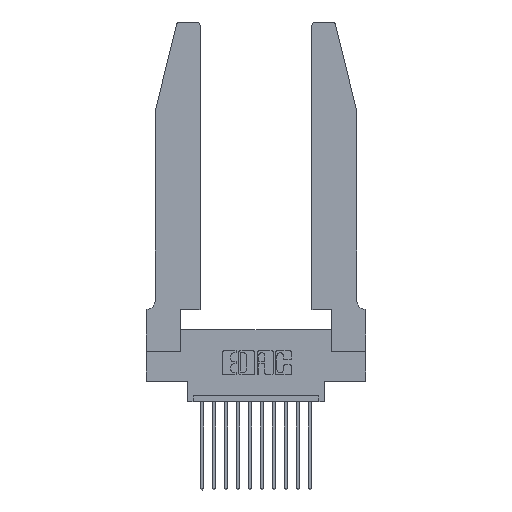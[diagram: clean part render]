
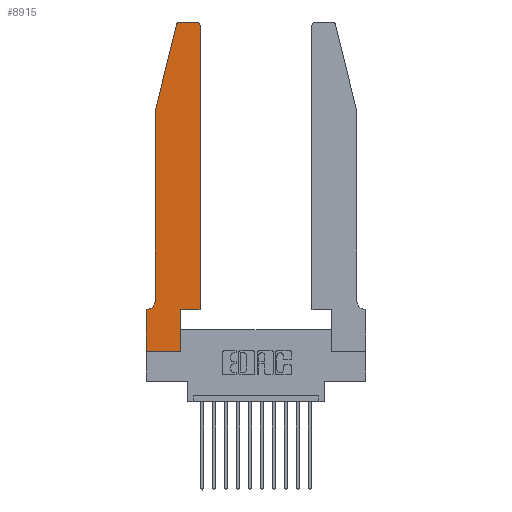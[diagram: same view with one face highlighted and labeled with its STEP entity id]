
A CAD part, top view. The second image highlights one B-rep face of the part: STEP entity #8915.
In plain terms, the highlighted planar face has unit normal (0, 0, 1).
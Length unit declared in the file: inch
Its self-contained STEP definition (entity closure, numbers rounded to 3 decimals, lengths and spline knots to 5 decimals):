
#252 = DIRECTION ( 'NONE',  ( 1., 0., 0. ) ) ;
#673 = VERTEX_POINT ( 'NONE', #13851 ) ;
#1145 = CARTESIAN_POINT ( 'NONE',  ( 0.25487, 2.72718, 0.37 ) ) ;
#1256 = CARTESIAN_POINT ( 'NONE',  ( 0.2865, 0.35, 0.37 ) ) ;
#1277 = DIRECTION ( 'NONE',  ( -1., 0., 0. ) ) ;
#1287 = CARTESIAN_POINT ( 'NONE',  ( 0.4505, 0.35, 0.37 ) ) ;
#1292 = EDGE_CURVE ( 'NONE', #7875, #4004, #4837, .T. ) ;
#1612 = CIRCLE ( 'NONE', #16716, 0.03 ) ;
#1732 = CARTESIAN_POINT ( 'NONE',  ( 0., 0.35, 0.37 ) ) ;
#1873 = VECTOR ( 'NONE', #9829, 39.37008 ) ;
#1878 = DIRECTION ( 'NONE',  ( 0., 0., 1. ) ) ;
#1887 = CARTESIAN_POINT ( 'NONE',  ( 0.284, 2.75, 0.37 ) ) ;
#2018 = VECTOR ( 'NONE', #13395, 39.37008 ) ;
#2041 = CARTESIAN_POINT ( 'NONE',  ( 0., 0.35, 0.37 ) ) ;
#2090 = VECTOR ( 'NONE', #2855, 39.37008 ) ;
#2194 = DIRECTION ( 'NONE',  ( -1., 0., 0. ) ) ;
#2246 = AXIS2_PLACEMENT_3D ( 'NONE', #15536, #1878, #14213 ) ;
#2300 = VERTEX_POINT ( 'NONE', #8853 ) ;
#2461 = VERTEX_POINT ( 'NONE', #11688 ) ;
#2654 = ORIENTED_EDGE ( 'NONE', *, *, #15632, .T. ) ;
#2749 = VECTOR ( 'NONE', #9596, 39.37008 ) ;
#2855 = DIRECTION ( 'NONE',  ( 1., 0., 0. ) ) ;
#2965 = EDGE_CURVE ( 'NONE', #9443, #16137, #1612, .T. ) ;
#3316 = CARTESIAN_POINT ( 'NONE',  ( 0.284, 2.72, 0.37 ) ) ;
#3427 = CARTESIAN_POINT ( 'NONE',  ( 0.0755, 2., 0.37 ) ) ;
#3888 = LINE ( 'NONE', #3427, #4703 ) ;
#4004 = VERTEX_POINT ( 'NONE', #6656 ) ;
#4189 = CARTESIAN_POINT ( 'NONE',  ( 0.0755, 2., 0.37 ) ) ;
#4335 = VERTEX_POINT ( 'NONE', #2041 ) ;
#4581 = EDGE_CURVE ( 'NONE', #13725, #2461, #10868, .T. ) ;
#4646 = CARTESIAN_POINT ( 'NONE',  ( 0.0755, 2., 0.37 ) ) ;
#4698 = DIRECTION ( 'NONE',  ( 0., 1., 0. ) ) ;
#4703 = VECTOR ( 'NONE', #10340, 39.37008 ) ;
#4837 = LINE ( 'NONE', #12212, #2018 ) ;
#4920 = ORIENTED_EDGE ( 'NONE', *, *, #13394, .T. ) ;
#5031 = VECTOR ( 'NONE', #9676, 39.37008 ) ;
#5240 = VERTEX_POINT ( 'NONE', #4189 ) ;
#5259 = AXIS2_PLACEMENT_3D ( 'NONE', #15546, #15660, #1277 ) ;
#5414 = LINE ( 'NONE', #12222, #5031 ) ;
#5914 = ORIENTED_EDGE ( 'NONE', *, *, #1292, .T. ) ;
#6072 = ORIENTED_EDGE ( 'NONE', *, *, #6856, .T. ) ;
#6265 = ORIENTED_EDGE ( 'NONE', *, *, #4581, .T. ) ;
#6473 = EDGE_CURVE ( 'NONE', #16137, #5240, #9374, .T. ) ;
#6656 = CARTESIAN_POINT ( 'NONE',  ( 0.2865, 0., 0.37 ) ) ;
#6856 = EDGE_CURVE ( 'NONE', #2300, #15438, #7971, .T. ) ;
#6866 = PLANE ( 'NONE',  #12857 ) ;
#7240 = CARTESIAN_POINT ( 'NONE',  ( 0., 0., 0.37 ) ) ;
#7875 = VERTEX_POINT ( 'NONE', #11843 ) ;
#7971 = CIRCLE ( 'NONE', #5259, 0.07 ) ;
#7999 = DIRECTION ( 'NONE',  ( 0., 0., 1. ) ) ;
#8172 = LINE ( 'NONE', #1256, #15443 ) ;
#8765 = LINE ( 'NONE', #7240, #1873 ) ;
#8788 = EDGE_LOOP ( 'NONE', ( #10304, #10822, #11894, #16695, #6072, #16342, #10317, #5914, #16578, #4920, #6265, #2654 ) ) ;
#8853 = CARTESIAN_POINT ( 'NONE',  ( 0.0755, 0.42, 0.37 ) ) ;
#8915 = ADVANCED_FACE ( 'NONE', ( #9703 ), #6866, .T. ) ;
#8918 = EDGE_CURVE ( 'NONE', #673, #9443, #5414, .T. ) ;
#9374 = LINE ( 'NONE', #4646, #12400 ) ;
#9443 = VERTEX_POINT ( 'NONE', #1887 ) ;
#9596 = DIRECTION ( 'NONE',  ( 0., 1., 0. ) ) ;
#9676 = DIRECTION ( 'NONE',  ( -1., 0., 0. ) ) ;
#9703 = FACE_OUTER_BOUND ( 'NONE', #8788, .T. ) ;
#9765 = VECTOR ( 'NONE', #2194, 39.37008 ) ;
#9829 = DIRECTION ( 'NONE',  ( 0., -1., 0. ) ) ;
#10304 = ORIENTED_EDGE ( 'NONE', *, *, #8918, .T. ) ;
#10317 = ORIENTED_EDGE ( 'NONE', *, *, #15269, .T. ) ;
#10340 = DIRECTION ( 'NONE',  ( 0., -1., 0. ) ) ;
#10822 = ORIENTED_EDGE ( 'NONE', *, *, #2965, .T. ) ;
#10868 = LINE ( 'NONE', #1287, #2749 ) ;
#11294 = CARTESIAN_POINT ( 'NONE',  ( 0.2865, 0.35, 0.37 ) ) ;
#11611 = VERTEX_POINT ( 'NONE', #11294 ) ;
#11688 = CARTESIAN_POINT ( 'NONE',  ( 0.4505, 2.72, 0.37 ) ) ;
#11843 = CARTESIAN_POINT ( 'NONE',  ( 0., 0., 0.37 ) ) ;
#11878 = CARTESIAN_POINT ( 'NONE',  ( 0.0055, 0.35, 0.37 ) ) ;
#11894 = ORIENTED_EDGE ( 'NONE', *, *, #6473, .T. ) ;
#12122 = CARTESIAN_POINT ( 'NONE',  ( 0.4505, 0.35, 0.37 ) ) ;
#12212 = CARTESIAN_POINT ( 'NONE',  ( 0., 0., 0.37 ) ) ;
#12222 = CARTESIAN_POINT ( 'NONE',  ( 0.2605, 2.75, 0.37 ) ) ;
#12400 = VECTOR ( 'NONE', #13676, 39.37008 ) ;
#12518 = CARTESIAN_POINT ( 'NONE',  ( 0.0755, 0.35, 0.37 ) ) ;
#12857 = AXIS2_PLACEMENT_3D ( 'NONE', #1732, #7999, #252 ) ;
#12892 = EDGE_CURVE ( 'NONE', #4004, #11611, #8172, .T. ) ;
#12946 = CIRCLE ( 'NONE', #2246, 0.03 ) ;
#13394 = EDGE_CURVE ( 'NONE', #11611, #13725, #15823, .T. ) ;
#13395 = DIRECTION ( 'NONE',  ( 1., 0., 0. ) ) ;
#13632 = EDGE_CURVE ( 'NONE', #5240, #2300, #3888, .T. ) ;
#13676 = DIRECTION ( 'NONE',  ( -0.239, -0.971, 0. ) ) ;
#13681 = EDGE_CURVE ( 'NONE', #15438, #4335, #13996, .T. ) ;
#13725 = VERTEX_POINT ( 'NONE', #16646 ) ;
#13851 = CARTESIAN_POINT ( 'NONE',  ( 0.4205, 2.75, 0.37 ) ) ;
#13996 = LINE ( 'NONE', #12518, #9765 ) ;
#14213 = DIRECTION ( 'NONE',  ( 1., 0., 0. ) ) ;
#14947 = DIRECTION ( 'NONE',  ( 0., 0., 1. ) ) ;
#15269 = EDGE_CURVE ( 'NONE', #4335, #7875, #8765, .T. ) ;
#15438 = VERTEX_POINT ( 'NONE', #11878 ) ;
#15443 = VECTOR ( 'NONE', #4698, 39.37008 ) ;
#15536 = CARTESIAN_POINT ( 'NONE',  ( 0.4205, 2.72, 0.37 ) ) ;
#15546 = CARTESIAN_POINT ( 'NONE',  ( 0.0055, 0.42, 0.37 ) ) ;
#15632 = EDGE_CURVE ( 'NONE', #2461, #673, #12946, .T. ) ;
#15660 = DIRECTION ( 'NONE',  ( 0., 0., -1. ) ) ;
#15823 = LINE ( 'NONE', #12122, #2090 ) ;
#16137 = VERTEX_POINT ( 'NONE', #1145 ) ;
#16196 = DIRECTION ( 'NONE',  ( 1., 0., 0. ) ) ;
#16342 = ORIENTED_EDGE ( 'NONE', *, *, #13681, .T. ) ;
#16578 = ORIENTED_EDGE ( 'NONE', *, *, #12892, .T. ) ;
#16646 = CARTESIAN_POINT ( 'NONE',  ( 0.4505, 0.35, 0.37 ) ) ;
#16695 = ORIENTED_EDGE ( 'NONE', *, *, #13632, .T. ) ;
#16716 = AXIS2_PLACEMENT_3D ( 'NONE', #3316, #14947, #16196 ) ;
